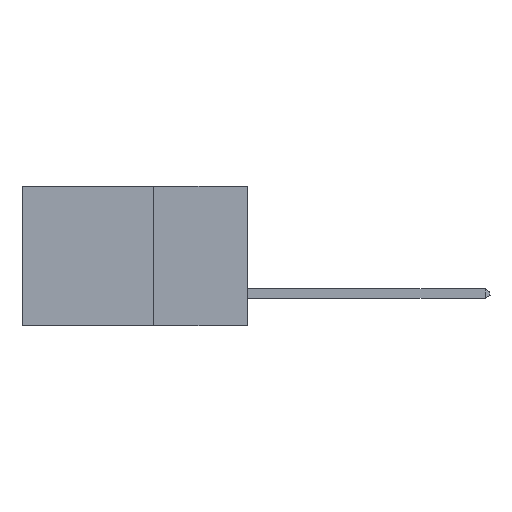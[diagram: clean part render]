
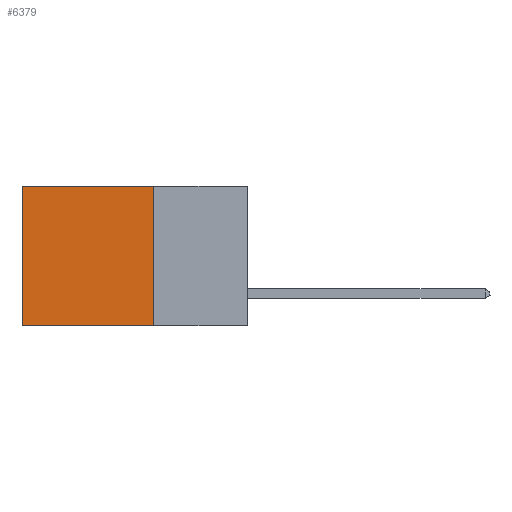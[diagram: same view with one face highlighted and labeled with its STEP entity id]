
A CAD part, left-side view. The second image highlights one B-rep face of the part: STEP entity #6379.
In plain terms, the highlighted planar face has unit normal (-1, 0, 0).
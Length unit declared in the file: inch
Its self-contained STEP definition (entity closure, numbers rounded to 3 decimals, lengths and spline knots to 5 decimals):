
#1163 = CARTESIAN_POINT ( 'NONE',  ( 0.298, 0.25, 0. ) ) ;
#1275 = LINE ( 'NONE', #21058, #8930 ) ;
#2117 = LINE ( 'NONE', #17548, #5811 ) ;
#3824 = LINE ( 'NONE', #23537, #24814 ) ;
#5004 = DIRECTION ( 'NONE',  ( 0., 0., -1. ) ) ;
#5811 = VECTOR ( 'NONE', #5004, 39.37008 ) ;
#6379 = ADVANCED_FACE ( 'NONE', ( #15504 ), #14114, .F. ) ;
#7566 = EDGE_CURVE ( 'NONE', #25025, #20340, #2117, .T. ) ;
#7619 = VECTOR ( 'NONE', #11532, 39.37008 ) ;
#8193 = EDGE_CURVE ( 'NONE', #18641, #25209, #13297, .T. ) ;
#8329 = DIRECTION ( 'NONE',  ( 0., 1., 0. ) ) ;
#8772 = ORIENTED_EDGE ( 'NONE', *, *, #9629, .T. ) ;
#8930 = VECTOR ( 'NONE', #8329, 39.37008 ) ;
#8960 = DIRECTION ( 'NONE',  ( 0., 1., 0. ) ) ;
#9455 = AXIS2_PLACEMENT_3D ( 'NONE', #18312, #9919, #24705 ) ;
#9629 = EDGE_CURVE ( 'NONE', #25025, #18641, #3824, .T. ) ;
#9919 = DIRECTION ( 'NONE',  ( 1., 0., 0. ) ) ;
#11354 = CARTESIAN_POINT ( 'NONE',  ( 0.298, 0.6, 0. ) ) ;
#11532 = DIRECTION ( 'NONE',  ( 0., 0., -1. ) ) ;
#13297 = LINE ( 'NONE', #11354, #7619 ) ;
#14114 = PLANE ( 'NONE',  #9455 ) ;
#14314 = CARTESIAN_POINT ( 'NONE',  ( 0.298, 0.6, 0. ) ) ;
#14381 = CARTESIAN_POINT ( 'NONE',  ( 0.298, 0.25, -0.37 ) ) ;
#15504 = FACE_OUTER_BOUND ( 'NONE', #24771, .T. ) ;
#17046 = CARTESIAN_POINT ( 'NONE',  ( 0.298, 0.6, -0.37 ) ) ;
#17548 = CARTESIAN_POINT ( 'NONE',  ( 0.298, 0.25, 0. ) ) ;
#18052 = ORIENTED_EDGE ( 'NONE', *, *, #8193, .T. ) ;
#18242 = ORIENTED_EDGE ( 'NONE', *, *, #23139, .F. ) ;
#18312 = CARTESIAN_POINT ( 'NONE',  ( 0.298, 0.25, 0. ) ) ;
#18641 = VERTEX_POINT ( 'NONE', #14314 ) ;
#20340 = VERTEX_POINT ( 'NONE', #14381 ) ;
#21058 = CARTESIAN_POINT ( 'NONE',  ( 0.298, 0.25, -0.37 ) ) ;
#23139 = EDGE_CURVE ( 'NONE', #20340, #25209, #1275, .T. ) ;
#23537 = CARTESIAN_POINT ( 'NONE',  ( 0.298, 0.25, 0. ) ) ;
#24705 = DIRECTION ( 'NONE',  ( 0., 0., -1. ) ) ;
#24771 = EDGE_LOOP ( 'NONE', ( #18052, #18242, #27136, #8772 ) ) ;
#24814 = VECTOR ( 'NONE', #8960, 39.37008 ) ;
#25025 = VERTEX_POINT ( 'NONE', #1163 ) ;
#25209 = VERTEX_POINT ( 'NONE', #17046 ) ;
#27136 = ORIENTED_EDGE ( 'NONE', *, *, #7566, .F. ) ;
